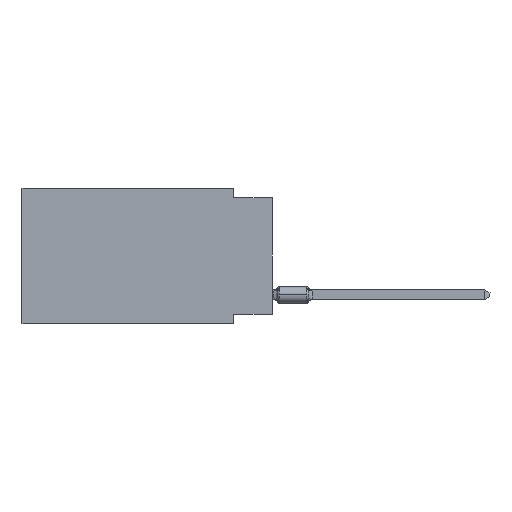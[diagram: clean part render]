
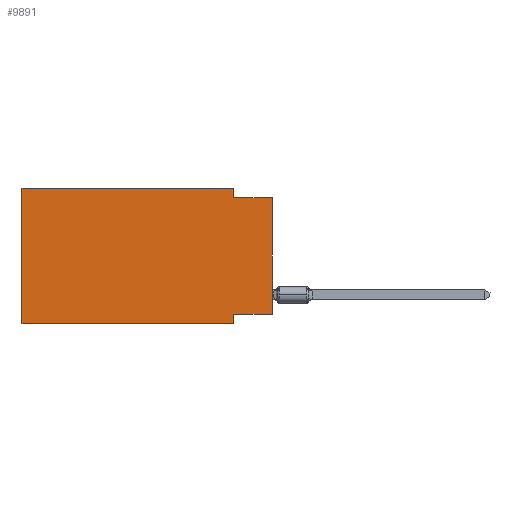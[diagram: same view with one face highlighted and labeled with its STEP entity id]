
A CAD part, left-side view. The second image highlights one B-rep face of the part: STEP entity #9891.
In plain terms, the highlighted planar face has unit normal (-1, 0, 0).
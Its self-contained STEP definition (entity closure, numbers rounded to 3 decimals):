
#25 = VERTEX_POINT ( 'NONE', #3045 ) ;
#146 = DIRECTION ( 'NONE',  ( 0., -1., 0. ) ) ;
#296 = EDGE_CURVE ( 'NONE', #22272, #26065, #9783, .T. ) ;
#1156 = LINE ( 'NONE', #25912, #15066 ) ;
#1709 = DIRECTION ( 'NONE',  ( 1., 0., 0. ) ) ;
#1851 = ORIENTED_EDGE ( 'NONE', *, *, #19805, .F. ) ;
#1854 = PLANE ( 'NONE',  #2313 ) ;
#2313 = AXIS2_PLACEMENT_3D ( 'NONE', #20803, #1709, #9119 ) ;
#2321 = DIRECTION ( 'NONE',  ( 0., -1., 0. ) ) ;
#2488 = CARTESIAN_POINT ( 'NONE',  ( 0., 2.54, -0.635 ) ) ;
#2508 = VECTOR ( 'NONE', #3979, 1000. ) ;
#2786 = DIRECTION ( 'NONE',  ( 0., 0., 1. ) ) ;
#3045 = CARTESIAN_POINT ( 'NONE',  ( 0., 16.383, 0. ) ) ;
#3099 = ORIENTED_EDGE ( 'NONE', *, *, #9959, .F. ) ;
#3176 = ORIENTED_EDGE ( 'NONE', *, *, #15182, .T. ) ;
#3362 = DIRECTION ( 'NONE',  ( 0., -1., 0. ) ) ;
#3535 = VECTOR ( 'NONE', #23725, 1000. ) ;
#3736 = ORIENTED_EDGE ( 'NONE', *, *, #23997, .F. ) ;
#3979 = DIRECTION ( 'NONE',  ( 0., 0., -1. ) ) ;
#4368 = VECTOR ( 'NONE', #146, 1000. ) ;
#4722 = DIRECTION ( 'NONE',  ( 0., 0., 1. ) ) ;
#4837 = CARTESIAN_POINT ( 'NONE',  ( 0., 16.383, -8.89 ) ) ;
#6835 = FACE_OUTER_BOUND ( 'NONE', #26703, .T. ) ;
#7320 = LINE ( 'NONE', #23550, #9267 ) ;
#7403 = DIRECTION ( 'NONE',  ( 0., 0., -1. ) ) ;
#9119 = DIRECTION ( 'NONE',  ( 0., 0., -1. ) ) ;
#9267 = VECTOR ( 'NONE', #2786, 1000. ) ;
#9628 = CARTESIAN_POINT ( 'NONE',  ( 0., 0., -8.255 ) ) ;
#9783 = LINE ( 'NONE', #9628, #3535 ) ;
#9891 = ADVANCED_FACE ( 'NONE', ( #6835 ), #1854, .F. ) ;
#9959 = EDGE_CURVE ( 'NONE', #23804, #25, #16247, .T. ) ;
#9999 = VECTOR ( 'NONE', #3362, 1000. ) ;
#11125 = CARTESIAN_POINT ( 'NONE',  ( 0., 16.383, 0. ) ) ;
#11821 = ORIENTED_EDGE ( 'NONE', *, *, #15905, .F. ) ;
#12846 = CARTESIAN_POINT ( 'NONE',  ( 0., 2.54, -8.89 ) ) ;
#13003 = VERTEX_POINT ( 'NONE', #18474 ) ;
#13045 = CARTESIAN_POINT ( 'NONE',  ( 0., 0., -0.635 ) ) ;
#13985 = LINE ( 'NONE', #11125, #16993 ) ;
#15066 = VECTOR ( 'NONE', #7403, 1000. ) ;
#15182 = EDGE_CURVE ( 'NONE', #22272, #13003, #7320, .T. ) ;
#15498 = LINE ( 'NONE', #24600, #2508 ) ;
#15875 = CARTESIAN_POINT ( 'NONE',  ( 0., 16.383, -8.89 ) ) ;
#15905 = EDGE_CURVE ( 'NONE', #26065, #22455, #1156, .T. ) ;
#16247 = LINE ( 'NONE', #25498, #24340 ) ;
#16393 = ORIENTED_EDGE ( 'NONE', *, *, #24374, .T. ) ;
#16449 = EDGE_CURVE ( 'NONE', #18027, #19130, #15498, .T. ) ;
#16993 = VECTOR ( 'NONE', #2321, 1000. ) ;
#18027 = VERTEX_POINT ( 'NONE', #25837 ) ;
#18344 = LINE ( 'NONE', #4837, #4368 ) ;
#18474 = CARTESIAN_POINT ( 'NONE',  ( 0., 0., -0.635 ) ) ;
#19130 = VERTEX_POINT ( 'NONE', #2488 ) ;
#19805 = EDGE_CURVE ( 'NONE', #19130, #13003, #24130, .T. ) ;
#20803 = CARTESIAN_POINT ( 'NONE',  ( 0., 16.383, 0. ) ) ;
#20940 = ORIENTED_EDGE ( 'NONE', *, *, #16449, .F. ) ;
#22272 = VERTEX_POINT ( 'NONE', #23775 ) ;
#22455 = VERTEX_POINT ( 'NONE', #12846 ) ;
#23550 = CARTESIAN_POINT ( 'NONE',  ( 0., 0., 0. ) ) ;
#23725 = DIRECTION ( 'NONE',  ( 0., 1., 0. ) ) ;
#23775 = CARTESIAN_POINT ( 'NONE',  ( 0., 0., -8.255 ) ) ;
#23804 = VERTEX_POINT ( 'NONE', #15875 ) ;
#23997 = EDGE_CURVE ( 'NONE', #25, #18027, #13985, .T. ) ;
#24130 = LINE ( 'NONE', #13045, #9999 ) ;
#24340 = VECTOR ( 'NONE', #4722, 1000. ) ;
#24374 = EDGE_CURVE ( 'NONE', #23804, #22455, #18344, .T. ) ;
#24600 = CARTESIAN_POINT ( 'NONE',  ( 0., 2.54, 0. ) ) ;
#25498 = CARTESIAN_POINT ( 'NONE',  ( 0., 16.383, 0. ) ) ;
#25837 = CARTESIAN_POINT ( 'NONE',  ( 0., 2.54, 0. ) ) ;
#25912 = CARTESIAN_POINT ( 'NONE',  ( 0., 2.54, -8.89 ) ) ;
#26065 = VERTEX_POINT ( 'NONE', #27725 ) ;
#26703 = EDGE_LOOP ( 'NONE', ( #3176, #1851, #20940, #3736, #3099, #16393, #11821, #28818 ) ) ;
#27725 = CARTESIAN_POINT ( 'NONE',  ( 0., 2.54, -8.255 ) ) ;
#28818 = ORIENTED_EDGE ( 'NONE', *, *, #296, .F. ) ;
